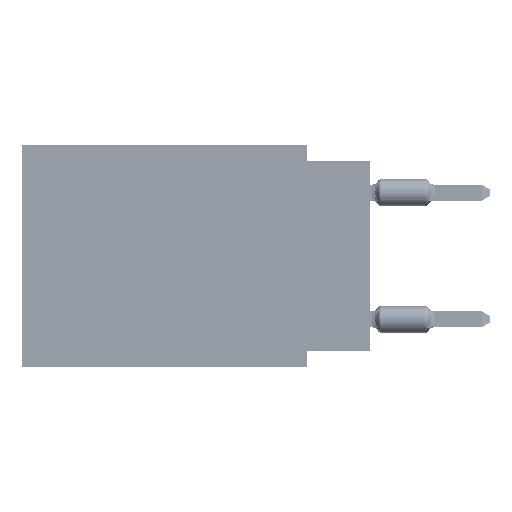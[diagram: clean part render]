
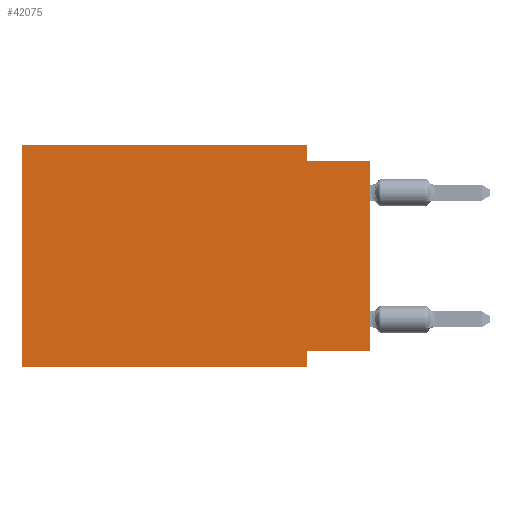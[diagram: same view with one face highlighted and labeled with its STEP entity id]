
A CAD part, left-side view. The second image highlights one B-rep face of the part: STEP entity #42075.
In plain terms, the highlighted planar face has unit normal (-1, 0, 0).
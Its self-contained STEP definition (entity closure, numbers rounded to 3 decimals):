
#404 = DIRECTION ( 'NONE',  ( 0., 1., 0. ) ) ;
#2828 = VERTEX_POINT ( 'NONE', #35011 ) ;
#5387 = AXIS2_PLACEMENT_3D ( 'NONE', #19668, #36078, #10687 ) ;
#5672 = CARTESIAN_POINT ( 'NONE',  ( 0., 13.97, 0. ) ) ;
#7847 = LINE ( 'NONE', #25350, #18767 ) ;
#9149 = EDGE_CURVE ( 'NONE', #64451, #27541, #7847, .T. ) ;
#9259 = LINE ( 'NONE', #31267, #42605 ) ;
#9929 = VECTOR ( 'NONE', #21845, 1000. ) ;
#10287 = EDGE_LOOP ( 'NONE', ( #64828, #30699, #24941, #51837, #68902, #17164, #56457, #43399 ) ) ;
#10687 = DIRECTION ( 'NONE',  ( 0., 0., -1. ) ) ;
#11774 = EDGE_CURVE ( 'NONE', #38203, #71568, #13238, .T. ) ;
#12260 = EDGE_CURVE ( 'NONE', #63993, #21281, #47031, .T. ) ;
#12416 = EDGE_CURVE ( 'NONE', #63993, #64451, #18609, .T. ) ;
#13238 = LINE ( 'NONE', #19558, #41689 ) ;
#13841 = CARTESIAN_POINT ( 'NONE',  ( 0., 0., -0.635 ) ) ;
#14831 = CARTESIAN_POINT ( 'NONE',  ( 0., 0., -0.635 ) ) ;
#16711 = DIRECTION ( 'NONE',  ( 0., -1., 0. ) ) ;
#17164 = ORIENTED_EDGE ( 'NONE', *, *, #56972, .T. ) ;
#18609 = LINE ( 'NONE', #57727, #19222 ) ;
#18767 = VECTOR ( 'NONE', #70771, 1000. ) ;
#19222 = VECTOR ( 'NONE', #404, 1000. ) ;
#19558 = CARTESIAN_POINT ( 'NONE',  ( 0., 13.97, 0. ) ) ;
#19638 = EDGE_CURVE ( 'NONE', #28391, #21281, #70477, .T. ) ;
#19668 = CARTESIAN_POINT ( 'NONE',  ( 0., 13.97, 0. ) ) ;
#21281 = VERTEX_POINT ( 'NONE', #14831 ) ;
#21845 = DIRECTION ( 'NONE',  ( 0., -1., 0. ) ) ;
#22081 = CARTESIAN_POINT ( 'NONE',  ( 0., 2.54, -8.255 ) ) ;
#23761 = LINE ( 'NONE', #63611, #67947 ) ;
#24523 = CARTESIAN_POINT ( 'NONE',  ( 0., 13.97, -8.89 ) ) ;
#24941 = ORIENTED_EDGE ( 'NONE', *, *, #69719, .F. ) ;
#25350 = CARTESIAN_POINT ( 'NONE',  ( 0., 2.54, -8.89 ) ) ;
#26699 = LINE ( 'NONE', #31896, #9929 ) ;
#27541 = VERTEX_POINT ( 'NONE', #41070 ) ;
#28391 = VERTEX_POINT ( 'NONE', #33881 ) ;
#28672 = VECTOR ( 'NONE', #46295, 1000. ) ;
#29486 = DIRECTION ( 'NONE',  ( 0., -1., 0. ) ) ;
#30699 = ORIENTED_EDGE ( 'NONE', *, *, #19638, .F. ) ;
#31267 = CARTESIAN_POINT ( 'NONE',  ( 0., 2.54, 0. ) ) ;
#31896 = CARTESIAN_POINT ( 'NONE',  ( 0., 13.97, 0. ) ) ;
#33881 = CARTESIAN_POINT ( 'NONE',  ( 0., 2.54, -0.635 ) ) ;
#35011 = CARTESIAN_POINT ( 'NONE',  ( 0., 2.54, 0. ) ) ;
#35566 = DIRECTION ( 'NONE',  ( 0., 0., 1. ) ) ;
#36078 = DIRECTION ( 'NONE',  ( 1., 0., 0. ) ) ;
#38203 = VERTEX_POINT ( 'NONE', #24523 ) ;
#41070 = CARTESIAN_POINT ( 'NONE',  ( 0., 2.54, -8.89 ) ) ;
#41689 = VECTOR ( 'NONE', #35566, 1000. ) ;
#42059 = DIRECTION ( 'NONE',  ( 0., 0., -1. ) ) ;
#42075 = ADVANCED_FACE ( 'NONE', ( #47987 ), #47227, .F. ) ;
#42605 = VECTOR ( 'NONE', #42059, 1000. ) ;
#43399 = ORIENTED_EDGE ( 'NONE', *, *, #12416, .F. ) ;
#46295 = DIRECTION ( 'NONE',  ( 0., 0., 1. ) ) ;
#47031 = LINE ( 'NONE', #69032, #28672 ) ;
#47227 = PLANE ( 'NONE',  #5387 ) ;
#47987 = FACE_OUTER_BOUND ( 'NONE', #10287, .T. ) ;
#51837 = ORIENTED_EDGE ( 'NONE', *, *, #59801, .F. ) ;
#56457 = ORIENTED_EDGE ( 'NONE', *, *, #9149, .F. ) ;
#56972 = EDGE_CURVE ( 'NONE', #38203, #27541, #23761, .T. ) ;
#57727 = CARTESIAN_POINT ( 'NONE',  ( 0., 0., -8.255 ) ) ;
#59426 = VECTOR ( 'NONE', #29486, 1000. ) ;
#59801 = EDGE_CURVE ( 'NONE', #71568, #2828, #26699, .T. ) ;
#63611 = CARTESIAN_POINT ( 'NONE',  ( 0., 13.97, -8.89 ) ) ;
#63993 = VERTEX_POINT ( 'NONE', #66902 ) ;
#64451 = VERTEX_POINT ( 'NONE', #22081 ) ;
#64828 = ORIENTED_EDGE ( 'NONE', *, *, #12260, .T. ) ;
#66902 = CARTESIAN_POINT ( 'NONE',  ( 0., 0., -8.255 ) ) ;
#67947 = VECTOR ( 'NONE', #16711, 1000. ) ;
#68902 = ORIENTED_EDGE ( 'NONE', *, *, #11774, .F. ) ;
#69032 = CARTESIAN_POINT ( 'NONE',  ( 0., 0., 0. ) ) ;
#69719 = EDGE_CURVE ( 'NONE', #2828, #28391, #9259, .T. ) ;
#70477 = LINE ( 'NONE', #13841, #59426 ) ;
#70771 = DIRECTION ( 'NONE',  ( 0., 0., -1. ) ) ;
#71568 = VERTEX_POINT ( 'NONE', #5672 ) ;
